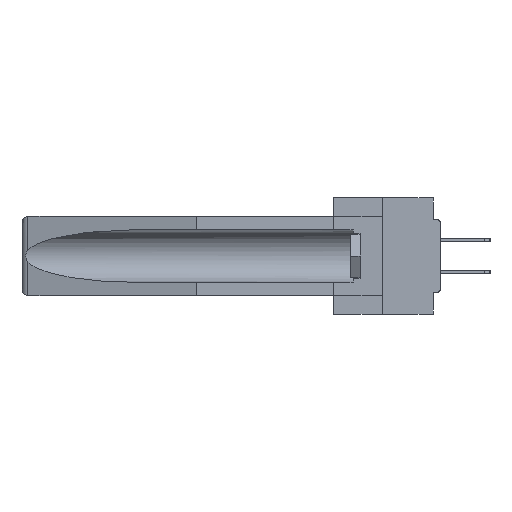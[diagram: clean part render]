
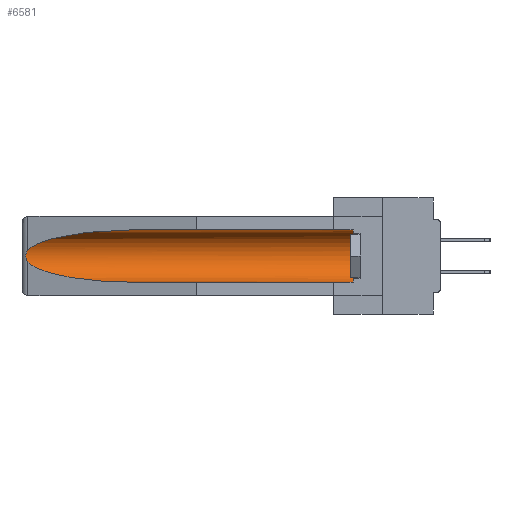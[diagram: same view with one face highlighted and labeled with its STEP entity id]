
A CAD part, left-side view. The second image highlights one B-rep face of the part: STEP entity #6581.
In plain terms, the highlighted cylindrical face has radius 2.857 mm (diameter 5.715 mm), a partial arc.
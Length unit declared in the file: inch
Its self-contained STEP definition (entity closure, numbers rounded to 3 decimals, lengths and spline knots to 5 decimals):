
#442 = CARTESIAN_POINT ( 'NONE',  ( 0.155, 1.07973, -0.059 ) ) ;
#1425 = CARTESIAN_POINT ( 'NONE',  ( 0.21114, 1.30732, -0.284 ) ) ;
#1433 = VERTEX_POINT ( 'NONE', #43623 ) ;
#1548 = VECTOR ( 'NONE', #2892, 39.37008 ) ;
#1667 = CARTESIAN_POINT ( 'NONE',  ( 0.26537, 1.52718, -0.19328 ) ) ;
#2367 =( BOUNDED_CURVE ( )  B_SPLINE_CURVE ( 3, ( #442, #2783, #42872, #11022 ),
 .UNSPECIFIED., .F., .F. ) 
 B_SPLINE_CURVE_WITH_KNOTS ( ( 4, 4 ),
 ( 4.71239, 6.08839 ),
 .UNSPECIFIED. ) 
 CURVE ( )  GEOMETRIC_REPRESENTATION_ITEM ( )  RATIONAL_B_SPLINE_CURVE ( ( 1., 0.848, 0.848, 1. ) ) 
 REPRESENTATION_ITEM ( '' )  );
#2783 = CARTESIAN_POINT ( 'NONE',  ( 0.21114, 1.30732, -0.059 ) ) ;
#2892 = DIRECTION ( 'NONE',  ( 0., 1., 0. ) ) ;
#3207 = CARTESIAN_POINT ( 'NONE',  ( 0.155, 0.126, -0.1715 ) ) ;
#3208 = EDGE_LOOP ( 'NONE', ( #14157, #4268, #34255, #42785, #21843, #36102 ) ) ;
#3538 = VERTEX_POINT ( 'NONE', #41971 ) ;
#4268 = ORIENTED_EDGE ( 'NONE', *, *, #36323, .T. ) ;
#6167 = DIRECTION ( 'NONE',  ( 0., 0., 1. ) ) ;
#6425 = CARTESIAN_POINT ( 'NONE',  ( 0.2673, 1.5327, -0.16383 ) ) ;
#6581 = ADVANCED_FACE ( 'NONE', ( #44465 ), #38939, .F. ) ;
#7055 = CARTESIAN_POINT ( 'NONE',  ( 0.26654, 1.53092, -0.15636 ) ) ;
#7256 = EDGE_CURVE ( 'NONE', #36450, #1433, #42248, .T. ) ;
#8001 = CARTESIAN_POINT ( 'NONE',  ( 0.26537, 1.52718, -0.19328 ) ) ;
#10626 = CARTESIAN_POINT ( 'NONE',  ( 0.26597, 1.52961, -0.15275 ) ) ;
#10646 = B_SPLINE_CURVE_WITH_KNOTS ( 'NONE', 3,
 ( #13896, #10626, #7055, #6425, #24754, #17614, #31810, #31205, #27825, #42307 ),
 .UNSPECIFIED., .F., .F.,
 ( 4, 2, 2, 2, 4 ),
 ( 0., 0.00029, 0.00058, 0.00087, 0.00117 ),
 .UNSPECIFIED. ) ;
#11022 = CARTESIAN_POINT ( 'NONE',  ( 0.26537, 1.52718, -0.14972 ) ) ;
#11382 = CARTESIAN_POINT ( 'NONE',  ( 0.155, 1.07973, -0.284 ) ) ;
#12947 = VECTOR ( 'NONE', #43674, 39.37008 ) ;
#13780 = DIRECTION ( 'NONE',  ( 0., 0., 1. ) ) ;
#13896 = CARTESIAN_POINT ( 'NONE',  ( 0.26537, 1.52718, -0.14972 ) ) ;
#14157 = ORIENTED_EDGE ( 'NONE', *, *, #40455, .T. ) ;
#17614 = CARTESIAN_POINT ( 'NONE',  ( 0.2675, 1.53308, -0.17534 ) ) ;
#20015 = CARTESIAN_POINT ( 'NONE',  ( 0.155, -0.30754, -0.1715 ) ) ;
#20312 = DIRECTION ( 'NONE',  ( 0., 1., 0. ) ) ;
#21843 = ORIENTED_EDGE ( 'NONE', *, *, #37900, .T. ) ;
#22940 = AXIS2_PLACEMENT_3D ( 'NONE', #20015, #20312, #6167 ) ;
#23763 =( BOUNDED_CURVE ( )  B_SPLINE_CURVE ( 3, ( #8001, #32888, #1425, #11382 ),
 .UNSPECIFIED., .F., .F. ) 
 B_SPLINE_CURVE_WITH_KNOTS ( ( 4, 4 ),
 ( 0.1948, 1.5708 ),
 .UNSPECIFIED. ) 
 CURVE ( )  GEOMETRIC_REPRESENTATION_ITEM ( )  RATIONAL_B_SPLINE_CURVE ( ( 1., 0.848, 0.848, 1. ) ) 
 REPRESENTATION_ITEM ( '' )  );
#24754 = CARTESIAN_POINT ( 'NONE',  ( 0.2675, 1.53308, -0.16763 ) ) ;
#26017 = VERTEX_POINT ( 'NONE', #1667 ) ;
#27825 = CARTESIAN_POINT ( 'NONE',  ( 0.26597, 1.5296, -0.19026 ) ) ;
#28975 = VERTEX_POINT ( 'NONE', #30949 ) ;
#29659 = CARTESIAN_POINT ( 'NONE',  ( 0.155, 1.07973, -0.284 ) ) ;
#30426 = CIRCLE ( 'NONE', #40260, 0.1125 ) ;
#30949 = CARTESIAN_POINT ( 'NONE',  ( 0.155, 0.126, -0.284 ) ) ;
#31205 = CARTESIAN_POINT ( 'NONE',  ( 0.26655, 1.53094, -0.18657 ) ) ;
#31810 = CARTESIAN_POINT ( 'NONE',  ( 0.2673, 1.53269, -0.17917 ) ) ;
#32888 = CARTESIAN_POINT ( 'NONE',  ( 0.25451, 1.48313, -0.24835 ) ) ;
#33491 = CARTESIAN_POINT ( 'NONE',  ( 0.155, -0.30754, -0.059 ) ) ;
#34255 = ORIENTED_EDGE ( 'NONE', *, *, #37720, .T. ) ;
#35932 = LINE ( 'NONE', #45286, #1548 ) ;
#36102 = ORIENTED_EDGE ( 'NONE', *, *, #7256, .T. ) ;
#36323 = EDGE_CURVE ( 'NONE', #3538, #26017, #10646, .T. ) ;
#36450 = VERTEX_POINT ( 'NONE', #40762 ) ;
#37720 = EDGE_CURVE ( 'NONE', #26017, #41799, #23763, .T. ) ;
#37900 = EDGE_CURVE ( 'NONE', #28975, #36450, #30426, .T. ) ;
#38674 = DIRECTION ( 'NONE',  ( 0., -1., 0. ) ) ;
#38939 = CYLINDRICAL_SURFACE ( 'NONE', #22940, 0.1125 ) ;
#40260 = AXIS2_PLACEMENT_3D ( 'NONE', #3207, #38674, #13780 ) ;
#40455 = EDGE_CURVE ( 'NONE', #1433, #3538, #2367, .T. ) ;
#40762 = CARTESIAN_POINT ( 'NONE',  ( 0.155, 0.126, -0.059 ) ) ;
#41799 = VERTEX_POINT ( 'NONE', #29659 ) ;
#41971 = CARTESIAN_POINT ( 'NONE',  ( 0.26537, 1.52718, -0.14972 ) ) ;
#42248 = LINE ( 'NONE', #33491, #12947 ) ;
#42307 = CARTESIAN_POINT ( 'NONE',  ( 0.26537, 1.52718, -0.19328 ) ) ;
#42785 = ORIENTED_EDGE ( 'NONE', *, *, #44832, .F. ) ;
#42872 = CARTESIAN_POINT ( 'NONE',  ( 0.25451, 1.48313, -0.09465 ) ) ;
#43623 = CARTESIAN_POINT ( 'NONE',  ( 0.155, 1.07973, -0.059 ) ) ;
#43674 = DIRECTION ( 'NONE',  ( 0., 1., 0. ) ) ;
#44465 = FACE_OUTER_BOUND ( 'NONE', #3208, .T. ) ;
#44832 = EDGE_CURVE ( 'NONE', #28975, #41799, #35932, .T. ) ;
#45286 = CARTESIAN_POINT ( 'NONE',  ( 0.155, -0.30754, -0.284 ) ) ;
